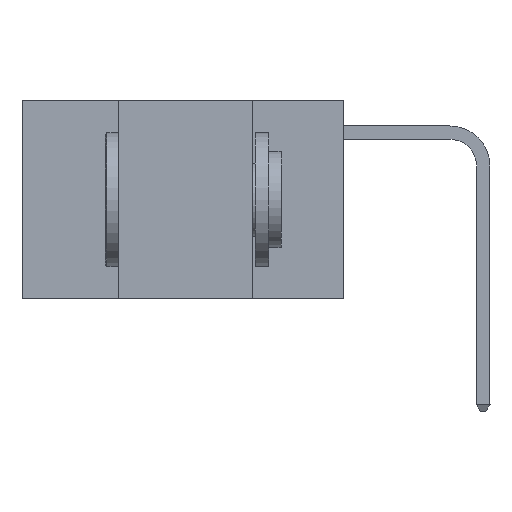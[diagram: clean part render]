
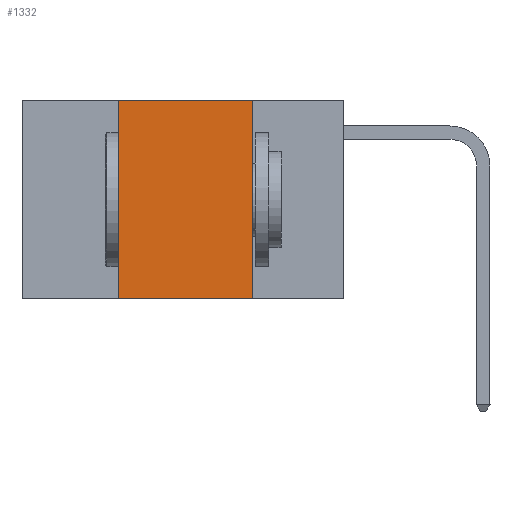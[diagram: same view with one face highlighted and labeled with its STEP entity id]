
A CAD part, left-side view. The second image highlights one B-rep face of the part: STEP entity #1332.
In plain terms, the highlighted planar face has unit normal (-1, 0, 0).
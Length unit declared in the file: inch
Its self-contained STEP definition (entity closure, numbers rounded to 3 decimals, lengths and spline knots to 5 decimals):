
#842 = EDGE_CURVE ( 'NONE', #9493, #14247, #6284, .T. ) ;
#1202 = EDGE_CURVE ( 'NONE', #9493, #15864, #3474, .T. ) ;
#1332 = ADVANCED_FACE ( 'NONE', ( #2443 ), #4888, .F. ) ;
#1524 = LINE ( 'NONE', #7200, #1609 ) ;
#1609 = VECTOR ( 'NONE', #7167, 39.37008 ) ;
#2443 = FACE_OUTER_BOUND ( 'NONE', #13401, .T. ) ;
#3254 = VECTOR ( 'NONE', #7286, 39.37008 ) ;
#3474 = LINE ( 'NONE', #7676, #3254 ) ;
#3600 = EDGE_CURVE ( 'NONE', #4139, #15864, #6468, .T. ) ;
#4124 = DIRECTION ( 'NONE',  ( 0., 0., -1. ) ) ;
#4139 = VERTEX_POINT ( 'NONE', #14251 ) ;
#4518 = CARTESIAN_POINT ( 'NONE',  ( 0., 0.17, 0. ) ) ;
#4721 = DIRECTION ( 'NONE',  ( 0., 0., -1. ) ) ;
#4867 = DIRECTION ( 'NONE',  ( 1., 0., 0. ) ) ;
#4888 = PLANE ( 'NONE',  #9708 ) ;
#5451 = CARTESIAN_POINT ( 'NONE',  ( 0., 0.6, 0. ) ) ;
#6011 = VECTOR ( 'NONE', #6261, 39.37008 ) ;
#6022 = CARTESIAN_POINT ( 'NONE',  ( 0., 0.42, 0. ) ) ;
#6261 = DIRECTION ( 'NONE',  ( 0., 0., 1. ) ) ;
#6284 = LINE ( 'NONE', #6022, #6011 ) ;
#6447 = VECTOR ( 'NONE', #4124, 39.37008 ) ;
#6468 = LINE ( 'NONE', #4518, #6447 ) ;
#7167 = DIRECTION ( 'NONE',  ( 0., -1., 0. ) ) ;
#7200 = CARTESIAN_POINT ( 'NONE',  ( 0., 0.6, 0. ) ) ;
#7233 = EDGE_CURVE ( 'NONE', #14247, #4139, #1524, .T. ) ;
#7286 = DIRECTION ( 'NONE',  ( 0., -1., 0. ) ) ;
#7676 = CARTESIAN_POINT ( 'NONE',  ( 0., 0.6, -0.37 ) ) ;
#9308 = CARTESIAN_POINT ( 'NONE',  ( 0., 0.42, 0. ) ) ;
#9493 = VERTEX_POINT ( 'NONE', #15888 ) ;
#9708 = AXIS2_PLACEMENT_3D ( 'NONE', #5451, #4867, #4721 ) ;
#12025 = ORIENTED_EDGE ( 'NONE', *, *, #3600, .F. ) ;
#12163 = ORIENTED_EDGE ( 'NONE', *, *, #7233, .F. ) ;
#12185 = ORIENTED_EDGE ( 'NONE', *, *, #842, .F. ) ;
#12382 = ORIENTED_EDGE ( 'NONE', *, *, #1202, .T. ) ;
#13401 = EDGE_LOOP ( 'NONE', ( #12025, #12163, #12185, #12382 ) ) ;
#14247 = VERTEX_POINT ( 'NONE', #9308 ) ;
#14251 = CARTESIAN_POINT ( 'NONE',  ( 0., 0.17, 0. ) ) ;
#14350 = CARTESIAN_POINT ( 'NONE',  ( 0., 0.17, -0.37 ) ) ;
#15864 = VERTEX_POINT ( 'NONE', #14350 ) ;
#15888 = CARTESIAN_POINT ( 'NONE',  ( 0., 0.42, -0.37 ) ) ;
